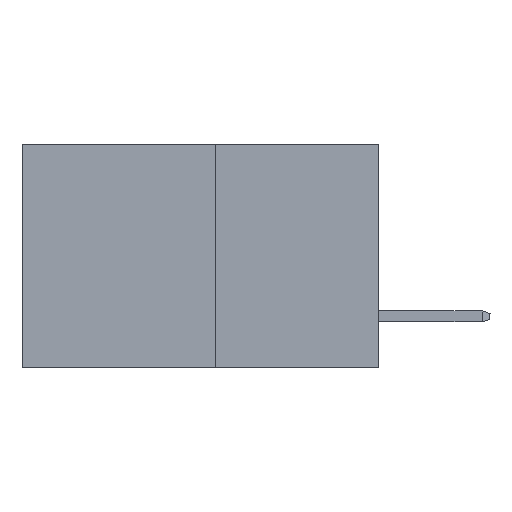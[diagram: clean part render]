
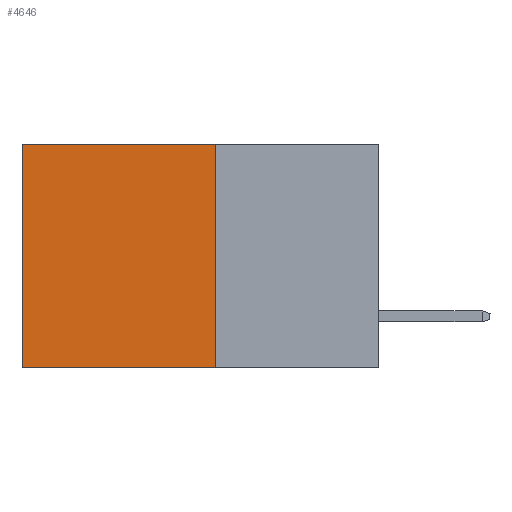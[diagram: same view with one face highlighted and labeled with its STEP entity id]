
A CAD part, left-side view. The second image highlights one B-rep face of the part: STEP entity #4646.
In plain terms, the highlighted planar face has unit normal (-1, 0, 0).
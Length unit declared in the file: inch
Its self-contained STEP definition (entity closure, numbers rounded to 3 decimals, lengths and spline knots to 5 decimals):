
#508 = LINE ( 'NONE', #8175, #10196 ) ;
#1237 = VERTEX_POINT ( 'NONE', #10976 ) ;
#1822 = CARTESIAN_POINT ( 'NONE',  ( 0.277, 0.27, -0.37 ) ) ;
#2357 = VECTOR ( 'NONE', #3862, 39.37008 ) ;
#2741 = DIRECTION ( 'NONE',  ( 0., 0., -1. ) ) ;
#2776 = EDGE_CURVE ( 'NONE', #7275, #1237, #7592, .T. ) ;
#3408 = EDGE_LOOP ( 'NONE', ( #7537, #8063, #8588, #5392 ) ) ;
#3862 = DIRECTION ( 'NONE',  ( 0., 1., 0. ) ) ;
#3911 = CARTESIAN_POINT ( 'NONE',  ( 0.277, 0.27, 0. ) ) ;
#4646 = ADVANCED_FACE ( 'NONE', ( #8397 ), #11347, .F. ) ;
#4754 = VECTOR ( 'NONE', #2741, 39.37008 ) ;
#5392 = ORIENTED_EDGE ( 'NONE', *, *, #7735, .T. ) ;
#5525 = CARTESIAN_POINT ( 'NONE',  ( 0.277, 0.59, -0.37 ) ) ;
#7275 = VERTEX_POINT ( 'NONE', #7432 ) ;
#7342 = AXIS2_PLACEMENT_3D ( 'NONE', #11219, #11002, #10992 ) ;
#7432 = CARTESIAN_POINT ( 'NONE',  ( 0.277, 0.27, 0. ) ) ;
#7472 = DIRECTION ( 'NONE',  ( 0., 1., 0. ) ) ;
#7537 = ORIENTED_EDGE ( 'NONE', *, *, #9339, .T. ) ;
#7592 = LINE ( 'NONE', #1822, #4754 ) ;
#7666 = CARTESIAN_POINT ( 'NONE',  ( 0.277, 0.27, -0.37 ) ) ;
#7735 = EDGE_CURVE ( 'NONE', #7275, #10621, #9838, .T. ) ;
#8063 = ORIENTED_EDGE ( 'NONE', *, *, #8822, .F. ) ;
#8175 = CARTESIAN_POINT ( 'NONE',  ( 0.277, 0.59, -0.37 ) ) ;
#8397 = FACE_OUTER_BOUND ( 'NONE', #3408, .T. ) ;
#8588 = ORIENTED_EDGE ( 'NONE', *, *, #2776, .F. ) ;
#8822 = EDGE_CURVE ( 'NONE', #1237, #8916, #9506, .T. ) ;
#8916 = VERTEX_POINT ( 'NONE', #5525 ) ;
#9085 = DIRECTION ( 'NONE',  ( 0., 0., -1. ) ) ;
#9242 = VECTOR ( 'NONE', #7472, 39.37008 ) ;
#9339 = EDGE_CURVE ( 'NONE', #10621, #8916, #508, .T. ) ;
#9506 = LINE ( 'NONE', #7666, #9242 ) ;
#9838 = LINE ( 'NONE', #3911, #2357 ) ;
#10196 = VECTOR ( 'NONE', #9085, 39.37008 ) ;
#10592 = CARTESIAN_POINT ( 'NONE',  ( 0.277, 0.59, 0. ) ) ;
#10621 = VERTEX_POINT ( 'NONE', #10592 ) ;
#10976 = CARTESIAN_POINT ( 'NONE',  ( 0.277, 0.27, -0.37 ) ) ;
#10992 = DIRECTION ( 'NONE',  ( 0., 0., -1. ) ) ;
#11002 = DIRECTION ( 'NONE',  ( 1., 0., 0. ) ) ;
#11219 = CARTESIAN_POINT ( 'NONE',  ( 0.277, 0.27, -0.37 ) ) ;
#11347 = PLANE ( 'NONE',  #7342 ) ;
